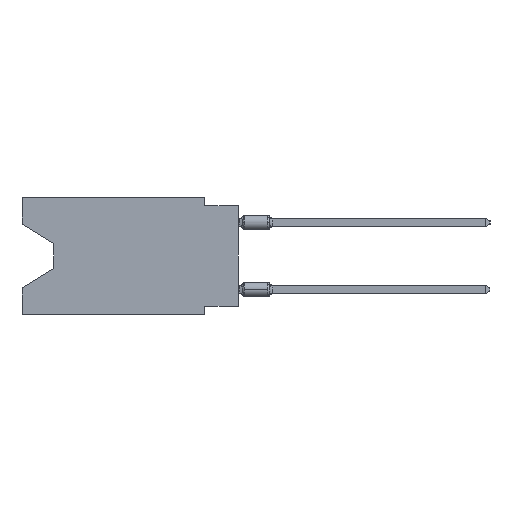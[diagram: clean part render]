
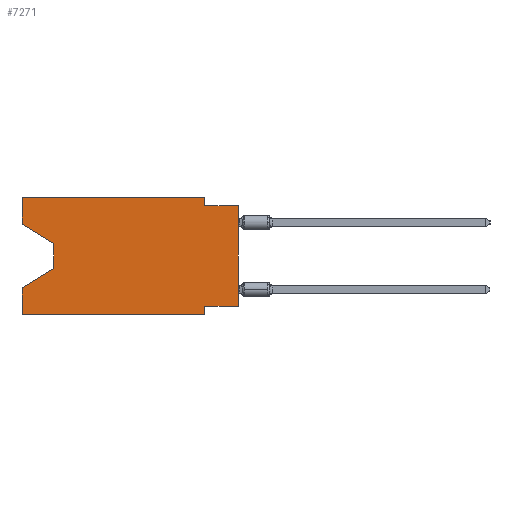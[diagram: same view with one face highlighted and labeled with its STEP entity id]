
A CAD part, left-side view. The second image highlights one B-rep face of the part: STEP entity #7271.
In plain terms, the highlighted planar face has unit normal (-1, 0, 0).
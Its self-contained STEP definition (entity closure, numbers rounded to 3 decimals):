
#316 = LINE ( 'NONE', #21081, #17551 ) ;
#679 = ORIENTED_EDGE ( 'NONE', *, *, #31026, .F. ) ;
#1028 = EDGE_CURVE ( 'NONE', #24943, #14048, #10977, .T. ) ;
#1065 = DIRECTION ( 'NONE',  ( 0., 1., 0. ) ) ;
#1256 = VECTOR ( 'NONE', #10899, 1000. ) ;
#1910 = DIRECTION ( 'NONE',  ( 0., 0., -1. ) ) ;
#2306 = VECTOR ( 'NONE', #27024, 1000. ) ;
#2411 = CARTESIAN_POINT ( 'NONE',  ( 0., 2.54, 0. ) ) ;
#2853 = ORIENTED_EDGE ( 'NONE', *, *, #11888, .T. ) ;
#3400 = CARTESIAN_POINT ( 'NONE',  ( 0., 2.54, -0.635 ) ) ;
#3651 = VECTOR ( 'NONE', #10477, 1000. ) ;
#3757 = LINE ( 'NONE', #11040, #30312 ) ;
#4951 = DIRECTION ( 'NONE',  ( 0., -1., 0. ) ) ;
#4964 = CARTESIAN_POINT ( 'NONE',  ( 0., 16.383, -2.038 ) ) ;
#5308 = CARTESIAN_POINT ( 'NONE',  ( 0., 0., -0.635 ) ) ;
#5528 = CARTESIAN_POINT ( 'NONE',  ( 0., 2.54, -8.89 ) ) ;
#5903 = EDGE_CURVE ( 'NONE', #25185, #23283, #7529, .T. ) ;
#5940 = ORIENTED_EDGE ( 'NONE', *, *, #26589, .F. ) ;
#6171 = LINE ( 'NONE', #21649, #24276 ) ;
#6600 = EDGE_CURVE ( 'NONE', #30011, #14723, #9379, .T. ) ;
#6686 = CARTESIAN_POINT ( 'NONE',  ( 0., 13.97, -5.385 ) ) ;
#6807 = FACE_OUTER_BOUND ( 'NONE', #26833, .T. ) ;
#7271 = ADVANCED_FACE ( 'NONE', ( #6807 ), #23796, .F. ) ;
#7306 = DIRECTION ( 'NONE',  ( 0., -0.855, -0.519 ) ) ;
#7529 = LINE ( 'NONE', #2411, #32483 ) ;
#8085 = EDGE_CURVE ( 'NONE', #24943, #29321, #3757, .T. ) ;
#8319 = CARTESIAN_POINT ( 'NONE',  ( 0., 16.383, 0. ) ) ;
#8483 = LINE ( 'NONE', #8319, #3651 ) ;
#8830 = ORIENTED_EDGE ( 'NONE', *, *, #22730, .T. ) ;
#8961 = DIRECTION ( 'NONE',  ( 1., 0., 0. ) ) ;
#9379 = LINE ( 'NONE', #16968, #2306 ) ;
#9491 = VECTOR ( 'NONE', #4951, 1000. ) ;
#9596 = CARTESIAN_POINT ( 'NONE',  ( 0., 16.383, -2.038 ) ) ;
#10194 = CARTESIAN_POINT ( 'NONE',  ( 0., 0., -0.635 ) ) ;
#10436 = CARTESIAN_POINT ( 'NONE',  ( 0., 16.383, -8.89 ) ) ;
#10477 = DIRECTION ( 'NONE',  ( 0., 0., 1. ) ) ;
#10549 = CARTESIAN_POINT ( 'NONE',  ( 0., 16.383, -6.852 ) ) ;
#10899 = DIRECTION ( 'NONE',  ( 0., 0., -1. ) ) ;
#10977 = LINE ( 'NONE', #13605, #11807 ) ;
#11040 = CARTESIAN_POINT ( 'NONE',  ( 0., 0., 0. ) ) ;
#11807 = VECTOR ( 'NONE', #1065, 1000. ) ;
#11887 = ORIENTED_EDGE ( 'NONE', *, *, #8085, .T. ) ;
#11888 = EDGE_CURVE ( 'NONE', #26571, #30011, #316, .T. ) ;
#13116 = CARTESIAN_POINT ( 'NONE',  ( 0., 0., -8.255 ) ) ;
#13605 = CARTESIAN_POINT ( 'NONE',  ( 0., 0., -8.255 ) ) ;
#13607 = VECTOR ( 'NONE', #7306, 1000. ) ;
#13758 = DIRECTION ( 'NONE',  ( 0., -1., 0. ) ) ;
#13829 = LINE ( 'NONE', #23407, #1256 ) ;
#13977 = DIRECTION ( 'NONE',  ( 0., 0., 1. ) ) ;
#14048 = VERTEX_POINT ( 'NONE', #28288 ) ;
#14137 = EDGE_CURVE ( 'NONE', #32532, #25185, #6171, .T. ) ;
#14189 = VECTOR ( 'NONE', #17589, 1000. ) ;
#14428 = VERTEX_POINT ( 'NONE', #10436 ) ;
#14723 = VERTEX_POINT ( 'NONE', #10549 ) ;
#15167 = ORIENTED_EDGE ( 'NONE', *, *, #6600, .T. ) ;
#15279 = VERTEX_POINT ( 'NONE', #4964 ) ;
#16968 = CARTESIAN_POINT ( 'NONE',  ( 0., 13.97, -5.385 ) ) ;
#17036 = DIRECTION ( 'NONE',  ( 0., 0., -1. ) ) ;
#17551 = VECTOR ( 'NONE', #30663, 1000. ) ;
#17589 = DIRECTION ( 'NONE',  ( 0., 0., 1. ) ) ;
#18128 = LINE ( 'NONE', #22904, #9491 ) ;
#18230 = LINE ( 'NONE', #30446, #14189 ) ;
#19213 = AXIS2_PLACEMENT_3D ( 'NONE', #26434, #8961, #17036 ) ;
#19411 = ORIENTED_EDGE ( 'NONE', *, *, #5903, .F. ) ;
#19487 = LINE ( 'NONE', #9596, #13607 ) ;
#19537 = ORIENTED_EDGE ( 'NONE', *, *, #20578, .T. ) ;
#20168 = CARTESIAN_POINT ( 'NONE',  ( 0., 2.54, 0. ) ) ;
#20578 = EDGE_CURVE ( 'NONE', #15279, #26571, #19487, .T. ) ;
#21081 = CARTESIAN_POINT ( 'NONE',  ( 0., 13.97, -3.505 ) ) ;
#21344 = VERTEX_POINT ( 'NONE', #5528 ) ;
#21649 = CARTESIAN_POINT ( 'NONE',  ( 0., 16.383, 0. ) ) ;
#22311 = ORIENTED_EDGE ( 'NONE', *, *, #23591, .F. ) ;
#22730 = EDGE_CURVE ( 'NONE', #14428, #21344, #18128, .T. ) ;
#22904 = CARTESIAN_POINT ( 'NONE',  ( 0., 16.383, -8.89 ) ) ;
#23283 = VERTEX_POINT ( 'NONE', #3400 ) ;
#23358 = LINE ( 'NONE', #10194, #24174 ) ;
#23407 = CARTESIAN_POINT ( 'NONE',  ( 0., 2.54, -8.89 ) ) ;
#23591 = EDGE_CURVE ( 'NONE', #14428, #14723, #8483, .T. ) ;
#23732 = CARTESIAN_POINT ( 'NONE',  ( 0., 13.97, -3.505 ) ) ;
#23796 = PLANE ( 'NONE',  #19213 ) ;
#24174 = VECTOR ( 'NONE', #25686, 1000. ) ;
#24276 = VECTOR ( 'NONE', #13758, 1000. ) ;
#24943 = VERTEX_POINT ( 'NONE', #13116 ) ;
#25185 = VERTEX_POINT ( 'NONE', #20168 ) ;
#25686 = DIRECTION ( 'NONE',  ( 0., -1., 0. ) ) ;
#26139 = CARTESIAN_POINT ( 'NONE',  ( 0., 16.383, 0. ) ) ;
#26434 = CARTESIAN_POINT ( 'NONE',  ( 0., 16.383, 0. ) ) ;
#26571 = VERTEX_POINT ( 'NONE', #23732 ) ;
#26589 = EDGE_CURVE ( 'NONE', #14048, #21344, #13829, .T. ) ;
#26833 = EDGE_LOOP ( 'NONE', ( #19537, #2853, #15167, #22311, #8830, #5940, #30527, #11887, #27783, #19411, #28135, #679 ) ) ;
#27024 = DIRECTION ( 'NONE',  ( 0., 0.855, -0.519 ) ) ;
#27783 = ORIENTED_EDGE ( 'NONE', *, *, #30593, .F. ) ;
#28135 = ORIENTED_EDGE ( 'NONE', *, *, #14137, .F. ) ;
#28288 = CARTESIAN_POINT ( 'NONE',  ( 0., 2.54, -8.255 ) ) ;
#29321 = VERTEX_POINT ( 'NONE', #5308 ) ;
#30011 = VERTEX_POINT ( 'NONE', #6686 ) ;
#30312 = VECTOR ( 'NONE', #13977, 1000. ) ;
#30446 = CARTESIAN_POINT ( 'NONE',  ( 0., 16.383, 0. ) ) ;
#30527 = ORIENTED_EDGE ( 'NONE', *, *, #1028, .F. ) ;
#30593 = EDGE_CURVE ( 'NONE', #23283, #29321, #23358, .T. ) ;
#30663 = DIRECTION ( 'NONE',  ( 0., 0., -1. ) ) ;
#31026 = EDGE_CURVE ( 'NONE', #15279, #32532, #18230, .T. ) ;
#32483 = VECTOR ( 'NONE', #1910, 1000. ) ;
#32532 = VERTEX_POINT ( 'NONE', #26139 ) ;
